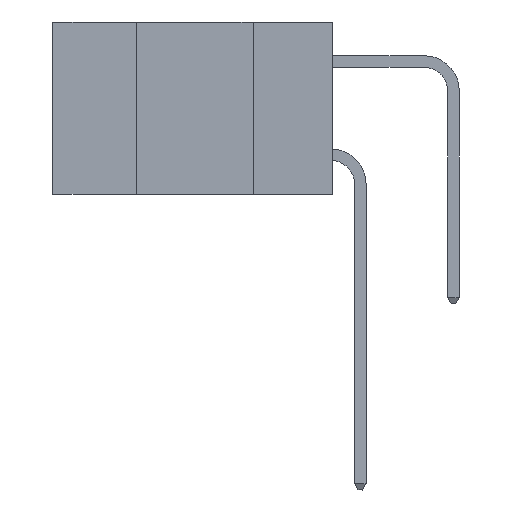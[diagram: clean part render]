
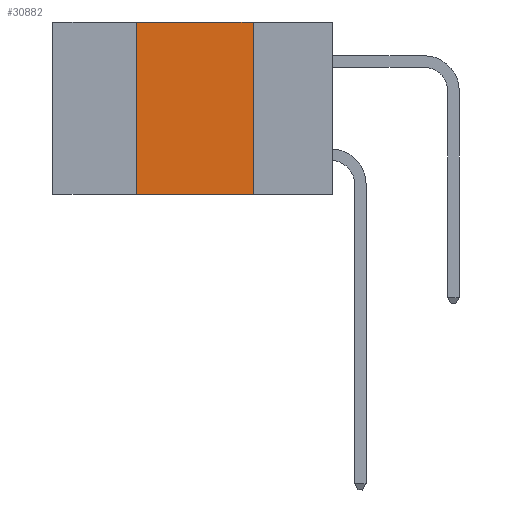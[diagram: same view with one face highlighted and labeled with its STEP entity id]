
A CAD part, left-side view. The second image highlights one B-rep face of the part: STEP entity #30882.
In plain terms, the highlighted planar face has unit normal (-1, 0, 0).
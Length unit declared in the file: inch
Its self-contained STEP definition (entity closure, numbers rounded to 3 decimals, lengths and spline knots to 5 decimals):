
#3147 = PLANE ( 'NONE',  #19937 ) ;
#4469 = ORIENTED_EDGE ( 'NONE', *, *, #22930, .F. ) ;
#5454 = LINE ( 'NONE', #33217, #25141 ) ;
#5747 = DIRECTION ( 'NONE',  ( 0., 0., -1. ) ) ;
#6681 = CARTESIAN_POINT ( 'NONE',  ( 0., 0.6, -0.37 ) ) ;
#11482 = VECTOR ( 'NONE', #32458, 39.37008 ) ;
#11909 = DIRECTION ( 'NONE',  ( 0., -1., 0. ) ) ;
#14352 = EDGE_CURVE ( 'NONE', #22994, #25015, #18366, .T. ) ;
#15985 = CARTESIAN_POINT ( 'NONE',  ( 0., 0.17, 0. ) ) ;
#16431 = CARTESIAN_POINT ( 'NONE',  ( 0., 0.17, -0.37 ) ) ;
#16627 = ORIENTED_EDGE ( 'NONE', *, *, #14352, .F. ) ;
#17198 = CARTESIAN_POINT ( 'NONE',  ( 0., 0.17, 0. ) ) ;
#18244 = ORIENTED_EDGE ( 'NONE', *, *, #24644, .T. ) ;
#18351 = CARTESIAN_POINT ( 'NONE',  ( 0., 0.42, 0. ) ) ;
#18366 = LINE ( 'NONE', #17198, #11482 ) ;
#19283 = LINE ( 'NONE', #6681, #31936 ) ;
#19937 = AXIS2_PLACEMENT_3D ( 'NONE', #26199, #21197, #5747 ) ;
#20603 = VERTEX_POINT ( 'NONE', #23101 ) ;
#20885 = DIRECTION ( 'NONE',  ( 0., 0., 1. ) ) ;
#21197 = DIRECTION ( 'NONE',  ( 1., 0., 0. ) ) ;
#21833 = EDGE_LOOP ( 'NONE', ( #16627, #23388, #4469, #18244 ) ) ;
#22930 = EDGE_CURVE ( 'NONE', #23003, #20603, #31292, .T. ) ;
#22994 = VERTEX_POINT ( 'NONE', #15985 ) ;
#23003 = VERTEX_POINT ( 'NONE', #23661 ) ;
#23101 = CARTESIAN_POINT ( 'NONE',  ( 0., 0.42, 0. ) ) ;
#23388 = ORIENTED_EDGE ( 'NONE', *, *, #27360, .F. ) ;
#23661 = CARTESIAN_POINT ( 'NONE',  ( 0., 0.42, -0.37 ) ) ;
#24101 = FACE_OUTER_BOUND ( 'NONE', #21833, .T. ) ;
#24644 = EDGE_CURVE ( 'NONE', #23003, #25015, #19283, .T. ) ;
#25015 = VERTEX_POINT ( 'NONE', #16431 ) ;
#25141 = VECTOR ( 'NONE', #28299, 39.37008 ) ;
#26199 = CARTESIAN_POINT ( 'NONE',  ( 0., 0.6, 0. ) ) ;
#27360 = EDGE_CURVE ( 'NONE', #20603, #22994, #5454, .T. ) ;
#28299 = DIRECTION ( 'NONE',  ( 0., -1., 0. ) ) ;
#30504 = VECTOR ( 'NONE', #20885, 39.37008 ) ;
#30882 = ADVANCED_FACE ( 'NONE', ( #24101 ), #3147, .F. ) ;
#31292 = LINE ( 'NONE', #18351, #30504 ) ;
#31936 = VECTOR ( 'NONE', #11909, 39.37008 ) ;
#32458 = DIRECTION ( 'NONE',  ( 0., 0., -1. ) ) ;
#33217 = CARTESIAN_POINT ( 'NONE',  ( 0., 0.6, 0. ) ) ;
